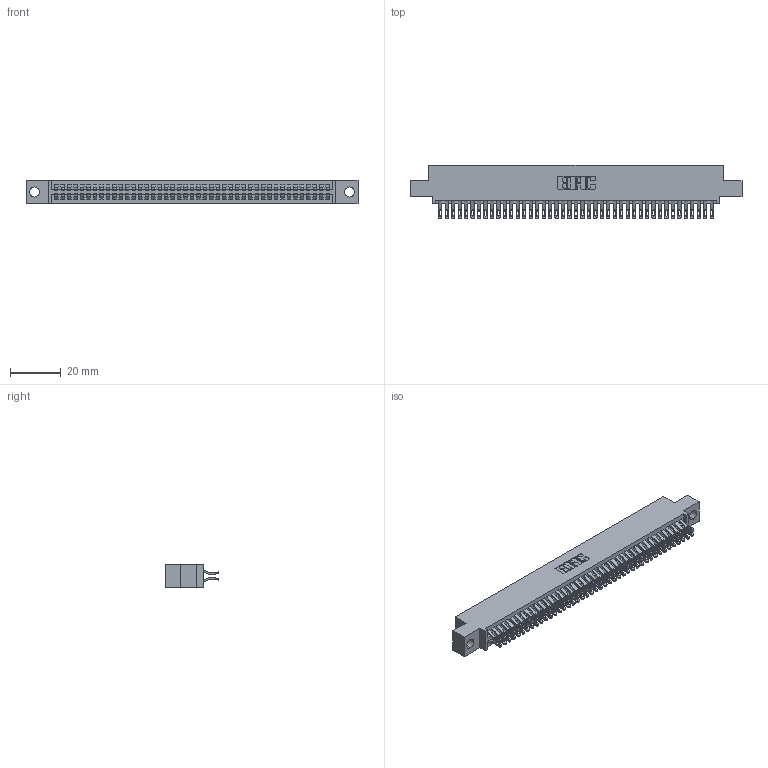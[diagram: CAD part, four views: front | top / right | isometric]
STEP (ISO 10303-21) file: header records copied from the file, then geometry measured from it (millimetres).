
FILE_DESCRIPTION (( 'STEP AP203' ), '1' );
FILE_NAME ('395-086-555-504.STEP', '2018-11-28T21:47:35', ( '' ), ( '' ), 'SwSTEP 2.0', 'SolidWorks 2016', '' );
FILE_SCHEMA (( 'CONFIG_CONTROL_DESIGN' ));
Length unit declared in the file: inch
Products named in the file (3): 345 Part_0.110 Offset - 0.156 Dia-TH; 395-086-555-504; 345-292-001_555 Tail
Assembly tree (87 placements, depth 2):
  395-086-555-504
    345 Part_0.110 Offset - 0.156 Dia-TH
    345-292-001_555 Tail  x86
Bounding box: 130.43 x 21.13 x 9.4 mm (x, y, z)
Volume: 12767.5 mm3; surface area: 19667.5 mm2
Topology: 87 solids, 87 shells, 4946 faces, 15575 edges, 10382 vertices
Faces by surface type: plane 2750, cylinder 2196
Entity records: 34065 total; most frequent: CARTESIAN_POINT 5746, ORIENTED_EDGE 5650, DIRECTION 5033, EDGE_CURVE 2825, VECTOR 2501, LINE 2501, VERTEX_POINT 1882, AXIS2_PLACEMENT_3D 1266
